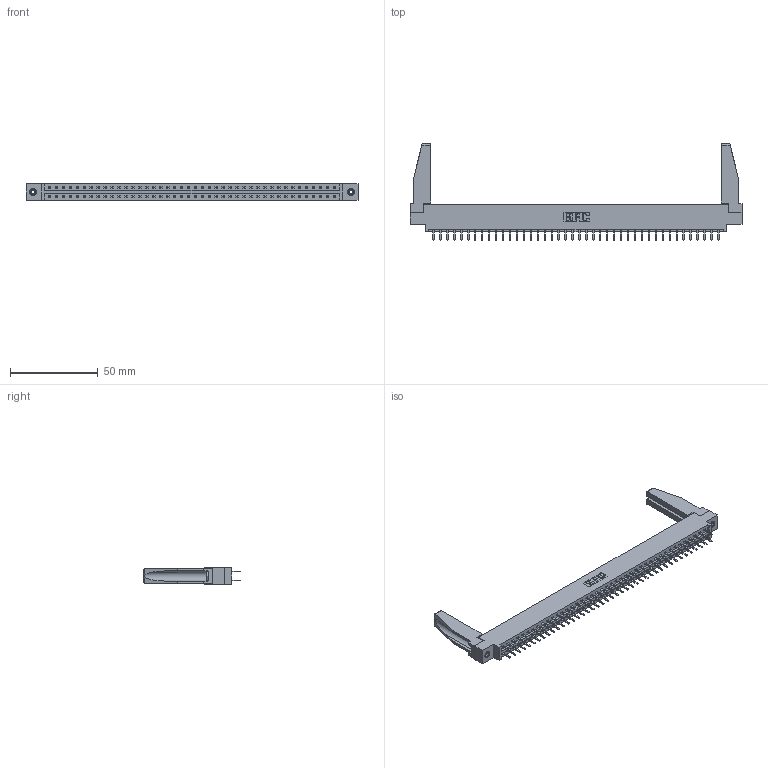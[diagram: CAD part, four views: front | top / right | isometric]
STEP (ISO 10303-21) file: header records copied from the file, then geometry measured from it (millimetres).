
FILE_DESCRIPTION (( 'STEP AP203' ), '1' );
FILE_NAME ('387-084-520-878.STEP', '2019-10-23T00:52:51', ( '' ), ( '' ), 'SwSTEP 2.0', 'SolidWorks 2016', '' );
FILE_SCHEMA (( 'CONFIG_CONTROL_DESIGN' ));
Length unit declared in the file: inch
Products named in the file (5): 345-292-001_345-293-120; 345-250-001_345-250-001-102; 387-084-520-878; 337 Part_0.170 Offset - 0.156 Dia-TI; 307-220-078
Assembly tree (89 placements, depth 2):
  387-084-520-878
    337 Part_0.170 Offset - 0.156 Dia-TI
    345-292-001_345-293-120  x84
    345-250-001_345-250-001-102  x2
    307-220-078  x2
Bounding box: 189.43 x 54.82 x 9.4 mm (x, y, z)
Volume: 23802.9 mm3; surface area: 26227.7 mm2
Topology: 89 solids, 89 shells, 5120 faces, 14849 edges, 9666 vertices
Faces by surface type: plane 3518, cylinder 1586, cone 12, torus 4
Entity records: 35250 total; most frequent: CARTESIAN_POINT 5952, ORIENTED_EDGE 5832, DIRECTION 5056, EDGE_CURVE 2916, LINE 2746, VECTOR 2746, VERTEX_POINT 1936, AXIS2_PLACEMENT_3D 1155
